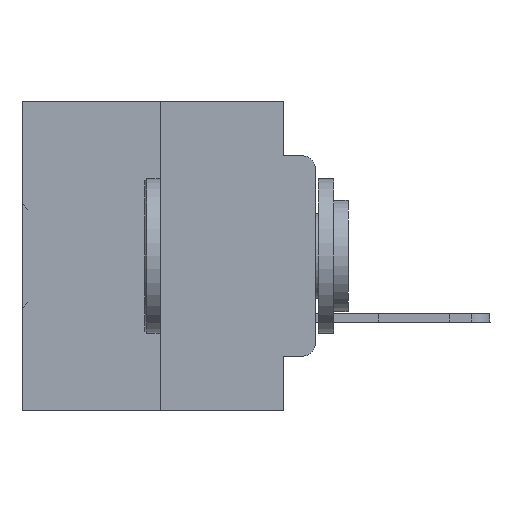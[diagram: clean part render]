
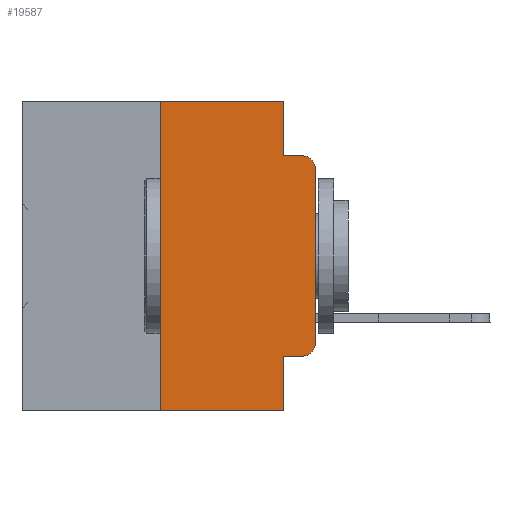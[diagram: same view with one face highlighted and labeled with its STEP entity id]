
A CAD part, left-side view. The second image highlights one B-rep face of the part: STEP entity #19587.
In plain terms, the highlighted planar face has unit normal (-1, 0, 0).
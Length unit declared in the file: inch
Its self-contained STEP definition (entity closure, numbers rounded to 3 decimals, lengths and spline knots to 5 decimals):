
#6 = ORIENTED_EDGE ( 'NONE', *, *, #22919, .T. ) ;
#1113 = CIRCLE ( 'NONE', #22768, 0.02 ) ;
#1389 = CARTESIAN_POINT ( 'NONE',  ( 0., 0.02, -0.4115 ) ) ;
#1531 = VERTEX_POINT ( 'NONE', #20993 ) ;
#1635 = DIRECTION ( 'NONE',  ( -1., 0., 0. ) ) ;
#1702 = CARTESIAN_POINT ( 'NONE',  ( 0., 0.051, -0.0885 ) ) ;
#2494 = DIRECTION ( 'NONE',  ( 0., 0., 1. ) ) ;
#3163 = LINE ( 'NONE', #11817, #34082 ) ;
#3241 = DIRECTION ( 'NONE',  ( 0., 0., -1. ) ) ;
#3269 = EDGE_CURVE ( 'NONE', #8861, #10880, #3762, .T. ) ;
#3356 = CARTESIAN_POINT ( 'NONE',  ( 0., 0., 0. ) ) ;
#3359 = LINE ( 'NONE', #3356, #13679 ) ;
#3579 = PLANE ( 'NONE',  #4309 ) ;
#3629 = CARTESIAN_POINT ( 'NONE',  ( 0., 0.051, -0.0885 ) ) ;
#3762 = LINE ( 'NONE', #1702, #20710 ) ;
#3808 = CIRCLE ( 'NONE', #18837, 0.02 ) ;
#4158 = EDGE_CURVE ( 'NONE', #17353, #25293, #29641, .T. ) ;
#4309 = AXIS2_PLACEMENT_3D ( 'NONE', #17938, #12804, #27082 ) ;
#4844 = CARTESIAN_POINT ( 'NONE',  ( 0., 0.02, -0.3915 ) ) ;
#5424 = EDGE_CURVE ( 'NONE', #29550, #18122, #13950, .T. ) ;
#6059 = ORIENTED_EDGE ( 'NONE', *, *, #5424, .F. ) ;
#6502 = VECTOR ( 'NONE', #2494, 39.37008 ) ;
#6506 = CARTESIAN_POINT ( 'NONE',  ( 0., 0.051, -0.4115 ) ) ;
#6955 = ORIENTED_EDGE ( 'NONE', *, *, #22235, .F. ) ;
#7090 = VECTOR ( 'NONE', #30393, 39.37008 ) ;
#8787 = VERTEX_POINT ( 'NONE', #35829 ) ;
#8861 = VERTEX_POINT ( 'NONE', #3629 ) ;
#9981 = ORIENTED_EDGE ( 'NONE', *, *, #31450, .F. ) ;
#10493 = EDGE_LOOP ( 'NONE', ( #34667, #21053, #21159, #6955, #6059, #33610, #6, #9981, #15617, #16191 ) ) ;
#10880 = VERTEX_POINT ( 'NONE', #24529 ) ;
#11817 = CARTESIAN_POINT ( 'NONE',  ( 0., 0.051, 0. ) ) ;
#12804 = DIRECTION ( 'NONE',  ( 1., 0., 0. ) ) ;
#13066 = VERTEX_POINT ( 'NONE', #23165 ) ;
#13679 = VECTOR ( 'NONE', #22920, 39.37008 ) ;
#13950 = LINE ( 'NONE', #16322, #16211 ) ;
#13999 = VERTEX_POINT ( 'NONE', #27453 ) ;
#14872 = EDGE_CURVE ( 'NONE', #1531, #29550, #26656, .T. ) ;
#15154 = EDGE_CURVE ( 'NONE', #25293, #13066, #3808, .T. ) ;
#15472 = DIRECTION ( 'NONE',  ( 0., -1., 0. ) ) ;
#15607 = LINE ( 'NONE', #22180, #7090 ) ;
#15617 = ORIENTED_EDGE ( 'NONE', *, *, #4158, .T. ) ;
#15673 = EDGE_CURVE ( 'NONE', #13999, #10880, #1113, .T. ) ;
#16061 = VECTOR ( 'NONE', #20092, 39.37008 ) ;
#16191 = ORIENTED_EDGE ( 'NONE', *, *, #15154, .T. ) ;
#16211 = VECTOR ( 'NONE', #33937, 39.37008 ) ;
#16322 = CARTESIAN_POINT ( 'NONE',  ( 0., 0.473, 0. ) ) ;
#16696 = VECTOR ( 'NONE', #15472, 39.37008 ) ;
#17353 = VERTEX_POINT ( 'NONE', #6506 ) ;
#17938 = CARTESIAN_POINT ( 'NONE',  ( 0., 0.473, 0. ) ) ;
#18122 = VERTEX_POINT ( 'NONE', #32536 ) ;
#18837 = AXIS2_PLACEMENT_3D ( 'NONE', #4844, #1635, #21534 ) ;
#19587 = ADVANCED_FACE ( 'NONE', ( #33421 ), #3579, .F. ) ;
#19759 = EDGE_CURVE ( 'NONE', #13066, #13999, #3359, .T. ) ;
#20092 = DIRECTION ( 'NONE',  ( 0., 0., -1. ) ) ;
#20710 = VECTOR ( 'NONE', #24631, 39.37008 ) ;
#20993 = CARTESIAN_POINT ( 'NONE',  ( 0., 0.25, -0.5 ) ) ;
#21053 = ORIENTED_EDGE ( 'NONE', *, *, #15673, .T. ) ;
#21159 = ORIENTED_EDGE ( 'NONE', *, *, #3269, .F. ) ;
#21534 = DIRECTION ( 'NONE',  ( 0., 0., -1. ) ) ;
#22180 = CARTESIAN_POINT ( 'NONE',  ( 0., 0.473, -0.5 ) ) ;
#22235 = EDGE_CURVE ( 'NONE', #18122, #8861, #33280, .T. ) ;
#22632 = CARTESIAN_POINT ( 'NONE',  ( 0., 0.25, 0. ) ) ;
#22768 = AXIS2_PLACEMENT_3D ( 'NONE', #25327, #28226, #35075 ) ;
#22919 = EDGE_CURVE ( 'NONE', #1531, #8787, #15607, .T. ) ;
#22920 = DIRECTION ( 'NONE',  ( 0., 0., 1. ) ) ;
#23165 = CARTESIAN_POINT ( 'NONE',  ( 0., 0., -0.3915 ) ) ;
#24529 = CARTESIAN_POINT ( 'NONE',  ( 0., 0.02, -0.0885 ) ) ;
#24631 = DIRECTION ( 'NONE',  ( 0., -1., 0. ) ) ;
#25293 = VERTEX_POINT ( 'NONE', #1389 ) ;
#25327 = CARTESIAN_POINT ( 'NONE',  ( 0., 0.02, -0.1085 ) ) ;
#25726 = CARTESIAN_POINT ( 'NONE',  ( 0., 0.051, 0. ) ) ;
#26656 = LINE ( 'NONE', #36855, #6502 ) ;
#26714 = CARTESIAN_POINT ( 'NONE',  ( 0., 0.051, -0.4115 ) ) ;
#27082 = DIRECTION ( 'NONE',  ( 0., 0., -1. ) ) ;
#27453 = CARTESIAN_POINT ( 'NONE',  ( 0., 0., -0.1085 ) ) ;
#28226 = DIRECTION ( 'NONE',  ( -1., 0., 0. ) ) ;
#29550 = VERTEX_POINT ( 'NONE', #22632 ) ;
#29641 = LINE ( 'NONE', #26714, #16696 ) ;
#30393 = DIRECTION ( 'NONE',  ( 0., -1., 0. ) ) ;
#31450 = EDGE_CURVE ( 'NONE', #17353, #8787, #3163, .T. ) ;
#32536 = CARTESIAN_POINT ( 'NONE',  ( 0., 0.051, 0. ) ) ;
#33280 = LINE ( 'NONE', #25726, #16061 ) ;
#33421 = FACE_OUTER_BOUND ( 'NONE', #10493, .T. ) ;
#33610 = ORIENTED_EDGE ( 'NONE', *, *, #14872, .F. ) ;
#33937 = DIRECTION ( 'NONE',  ( 0., -1., 0. ) ) ;
#34082 = VECTOR ( 'NONE', #3241, 39.37008 ) ;
#34667 = ORIENTED_EDGE ( 'NONE', *, *, #19759, .T. ) ;
#35075 = DIRECTION ( 'NONE',  ( 0., 0., -1. ) ) ;
#35829 = CARTESIAN_POINT ( 'NONE',  ( 0., 0.051, -0.5 ) ) ;
#36855 = CARTESIAN_POINT ( 'NONE',  ( 0., 0.25, 0. ) ) ;
